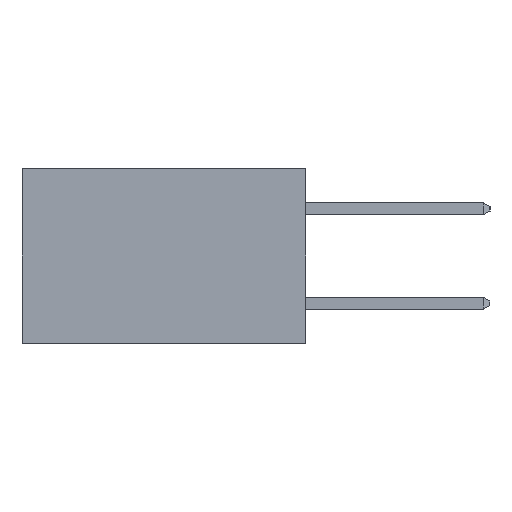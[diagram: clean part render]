
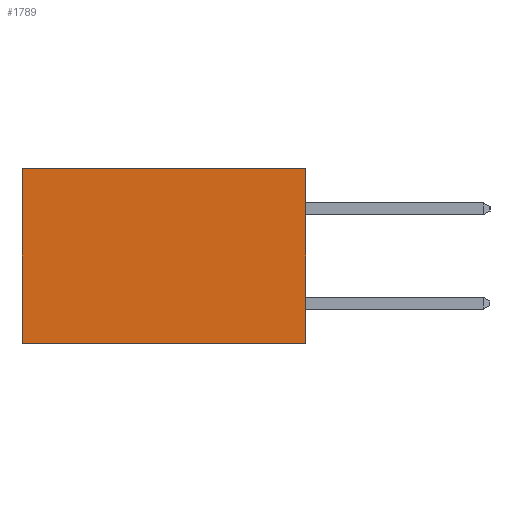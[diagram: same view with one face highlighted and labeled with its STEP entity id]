
A CAD part, left-side view. The second image highlights one B-rep face of the part: STEP entity #1789.
In plain terms, the highlighted planar face has unit normal (-1, 0, 0).
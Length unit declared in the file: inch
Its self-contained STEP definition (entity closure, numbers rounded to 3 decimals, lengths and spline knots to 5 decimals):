
#1167 = EDGE_CURVE ( 'NONE', #12285, #7700, #23203, .T. ) ;
#1526 = EDGE_CURVE ( 'NONE', #13862, #17972, #10409, .T. ) ;
#1789 = ADVANCED_FACE ( 'NONE', ( #13780 ), #4693, .F. ) ;
#2218 = CARTESIAN_POINT ( 'NONE',  ( 0.298, 0., 0. ) ) ;
#4520 = DIRECTION ( 'NONE',  ( 0., 0., -1. ) ) ;
#4693 = PLANE ( 'NONE',  #12700 ) ;
#4764 = VECTOR ( 'NONE', #4520, 39.37008 ) ;
#4840 = ORIENTED_EDGE ( 'NONE', *, *, #7073, .F. ) ;
#6451 = EDGE_CURVE ( 'NONE', #12285, #13862, #15054, .T. ) ;
#6709 = ORIENTED_EDGE ( 'NONE', *, *, #6451, .T. ) ;
#7073 = EDGE_CURVE ( 'NONE', #7700, #17972, #17272, .T. ) ;
#7483 = CARTESIAN_POINT ( 'NONE',  ( 0.298, 0., 0. ) ) ;
#7700 = VERTEX_POINT ( 'NONE', #8572 ) ;
#8572 = CARTESIAN_POINT ( 'NONE',  ( 0.298, 0., -0.37 ) ) ;
#8611 = ORIENTED_EDGE ( 'NONE', *, *, #1167, .F. ) ;
#10232 = VECTOR ( 'NONE', #15176, 39.37008 ) ;
#10409 = LINE ( 'NONE', #22796, #19394 ) ;
#10797 = CARTESIAN_POINT ( 'NONE',  ( 0.298, 0., -0.37 ) ) ;
#10914 = CARTESIAN_POINT ( 'NONE',  ( 0.298, 0.6, -0.37 ) ) ;
#11880 = CARTESIAN_POINT ( 'NONE',  ( 0.298, 0., 0. ) ) ;
#12285 = VERTEX_POINT ( 'NONE', #2218 ) ;
#12700 = AXIS2_PLACEMENT_3D ( 'NONE', #11880, #22870, #20096 ) ;
#13780 = FACE_OUTER_BOUND ( 'NONE', #16793, .T. ) ;
#13862 = VERTEX_POINT ( 'NONE', #13896 ) ;
#13896 = CARTESIAN_POINT ( 'NONE',  ( 0.298, 0.6, 0. ) ) ;
#14977 = CARTESIAN_POINT ( 'NONE',  ( 0.298, 0., 0. ) ) ;
#15054 = LINE ( 'NONE', #7483, #10232 ) ;
#15176 = DIRECTION ( 'NONE',  ( 0., 1., 0. ) ) ;
#15350 = ORIENTED_EDGE ( 'NONE', *, *, #1526, .T. ) ;
#16793 = EDGE_LOOP ( 'NONE', ( #15350, #4840, #8611, #6709 ) ) ;
#17272 = LINE ( 'NONE', #10797, #21914 ) ;
#17972 = VERTEX_POINT ( 'NONE', #10914 ) ;
#18044 = DIRECTION ( 'NONE',  ( 0., 1., 0. ) ) ;
#19374 = DIRECTION ( 'NONE',  ( 0., 0., -1. ) ) ;
#19394 = VECTOR ( 'NONE', #19374, 39.37008 ) ;
#20096 = DIRECTION ( 'NONE',  ( 0., 0., -1. ) ) ;
#21914 = VECTOR ( 'NONE', #18044, 39.37008 ) ;
#22796 = CARTESIAN_POINT ( 'NONE',  ( 0.298, 0.6, 0. ) ) ;
#22870 = DIRECTION ( 'NONE',  ( 1., 0., 0. ) ) ;
#23203 = LINE ( 'NONE', #14977, #4764 ) ;
